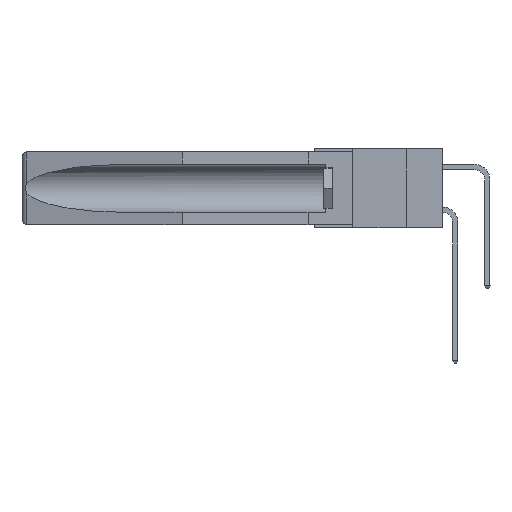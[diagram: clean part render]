
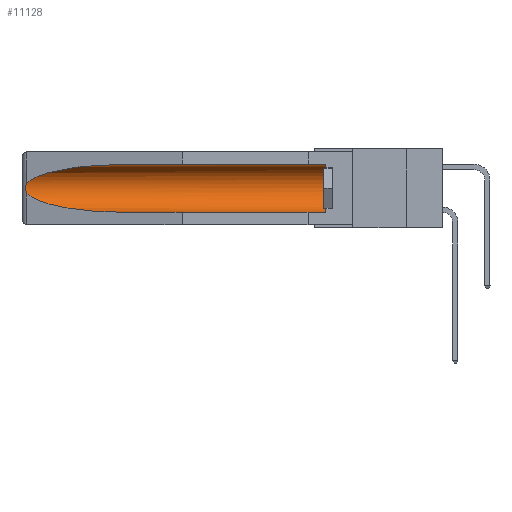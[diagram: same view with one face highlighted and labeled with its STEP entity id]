
A CAD part, left-side view. The second image highlights one B-rep face of the part: STEP entity #11128.
In plain terms, the highlighted cylindrical face has radius 2.857 mm (diameter 5.715 mm), a partial arc.
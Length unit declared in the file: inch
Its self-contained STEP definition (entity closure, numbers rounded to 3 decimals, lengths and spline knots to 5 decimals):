
#274 = DIRECTION ( 'NONE',  ( 0., 1., 0. ) ) ;
#505 = CARTESIAN_POINT ( 'NONE',  ( 0.26654, 1.53092, -0.15636 ) ) ;
#979 = CARTESIAN_POINT ( 'NONE',  ( 0.155, 1.07973, -0.059 ) ) ;
#1048 = ORIENTED_EDGE ( 'NONE', *, *, #12616, .F. ) ;
#1132 = CARTESIAN_POINT ( 'NONE',  ( 0.26597, 1.5296, -0.19026 ) ) ;
#1247 = CARTESIAN_POINT ( 'NONE',  ( 0.25451, 1.48313, -0.09465 ) ) ;
#1289 = DIRECTION ( 'NONE',  ( 0., 1., 0. ) ) ;
#1413 = CARTESIAN_POINT ( 'NONE',  ( 0.26537, 1.52718, -0.19328 ) ) ;
#1963 = B_SPLINE_CURVE_WITH_KNOTS ( 'NONE', 3,
 ( #6888, #18015, #505, #19783, #10522, #9368, #10989, #17308, #1132, #1413 ),
 .UNSPECIFIED., .F., .F.,
 ( 4, 2, 2, 2, 4 ),
 ( 0., 0.00029, 0.00058, 0.00087, 0.00117 ),
 .UNSPECIFIED. ) ;
#1995 = VERTEX_POINT ( 'NONE', #18974 ) ;
#2083 = EDGE_CURVE ( 'NONE', #9188, #8213, #16844, .T. ) ;
#2129 = CARTESIAN_POINT ( 'NONE',  ( 0.155, 1.07973, -0.284 ) ) ;
#3179 = EDGE_CURVE ( 'NONE', #16438, #1995, #3312, .T. ) ;
#3312 = CIRCLE ( 'NONE', #11565, 0.1125 ) ;
#3377 = CARTESIAN_POINT ( 'NONE',  ( 0.155, -0.30754, -0.1715 ) ) ;
#3535 = CARTESIAN_POINT ( 'NONE',  ( 0.21114, 1.30732, -0.284 ) ) ;
#3674 = CARTESIAN_POINT ( 'NONE',  ( 0.26537, 1.52718, -0.19328 ) ) ;
#5363 = LINE ( 'NONE', #9934, #17664 ) ;
#6613 = ORIENTED_EDGE ( 'NONE', *, *, #2083, .T. ) ;
#6749 = CYLINDRICAL_SURFACE ( 'NONE', #13404, 0.1125 ) ;
#6888 = CARTESIAN_POINT ( 'NONE',  ( 0.26537, 1.52718, -0.14972 ) ) ;
#6999 = EDGE_CURVE ( 'NONE', #15827, #7365, #18408, .T. ) ;
#7365 = VERTEX_POINT ( 'NONE', #19484 ) ;
#7812 = CARTESIAN_POINT ( 'NONE',  ( 0.155, 0.126, -0.1715 ) ) ;
#7888 = DIRECTION ( 'NONE',  ( 0., -1., 0. ) ) ;
#8213 = VERTEX_POINT ( 'NONE', #15224 ) ;
#8475 = FACE_OUTER_BOUND ( 'NONE', #11126, .T. ) ;
#8917 = CARTESIAN_POINT ( 'NONE',  ( 0.155, 0.126, -0.284 ) ) ;
#9064 = ORIENTED_EDGE ( 'NONE', *, *, #6999, .T. ) ;
#9072 = CARTESIAN_POINT ( 'NONE',  ( 0.21114, 1.30732, -0.059 ) ) ;
#9118 = CARTESIAN_POINT ( 'NONE',  ( 0.155, -0.30754, -0.284 ) ) ;
#9188 = VERTEX_POINT ( 'NONE', #16502 ) ;
#9368 = CARTESIAN_POINT ( 'NONE',  ( 0.2675, 1.53308, -0.17534 ) ) ;
#9403 = ORIENTED_EDGE ( 'NONE', *, *, #3179, .T. ) ;
#9411 = DIRECTION ( 'NONE',  ( 0., 0., 1. ) ) ;
#9858 = ORIENTED_EDGE ( 'NONE', *, *, #10091, .T. ) ;
#9934 = CARTESIAN_POINT ( 'NONE',  ( 0.155, -0.30754, -0.059 ) ) ;
#10091 = EDGE_CURVE ( 'NONE', #7365, #9188, #1963, .T. ) ;
#10522 = CARTESIAN_POINT ( 'NONE',  ( 0.2675, 1.53308, -0.16763 ) ) ;
#10989 = CARTESIAN_POINT ( 'NONE',  ( 0.2673, 1.53269, -0.17917 ) ) ;
#11126 = EDGE_LOOP ( 'NONE', ( #9064, #9858, #6613, #1048, #9403, #17494 ) ) ;
#11128 = ADVANCED_FACE ( 'NONE', ( #8475 ), #6749, .F. ) ;
#11535 = DIRECTION ( 'NONE',  ( 0., 1., 0. ) ) ;
#11565 = AXIS2_PLACEMENT_3D ( 'NONE', #7812, #7888, #9411 ) ;
#11685 = CARTESIAN_POINT ( 'NONE',  ( 0.25451, 1.48313, -0.24835 ) ) ;
#12213 = CARTESIAN_POINT ( 'NONE',  ( 0.26537, 1.52718, -0.14972 ) ) ;
#12616 = EDGE_CURVE ( 'NONE', #16438, #8213, #19848, .T. ) ;
#13202 = DIRECTION ( 'NONE',  ( 0., 0., 1. ) ) ;
#13235 = EDGE_CURVE ( 'NONE', #1995, #15827, #5363, .T. ) ;
#13404 = AXIS2_PLACEMENT_3D ( 'NONE', #3377, #274, #13202 ) ;
#15224 = CARTESIAN_POINT ( 'NONE',  ( 0.155, 1.07973, -0.284 ) ) ;
#15322 = VECTOR ( 'NONE', #1289, 39.37008 ) ;
#15827 = VERTEX_POINT ( 'NONE', #15912 ) ;
#15912 = CARTESIAN_POINT ( 'NONE',  ( 0.155, 1.07973, -0.059 ) ) ;
#16438 = VERTEX_POINT ( 'NONE', #8917 ) ;
#16502 = CARTESIAN_POINT ( 'NONE',  ( 0.26537, 1.52718, -0.19328 ) ) ;
#16844 =( BOUNDED_CURVE ( )  B_SPLINE_CURVE ( 3, ( #3674, #11685, #3535, #2129 ),
 .UNSPECIFIED., .F., .F. ) 
 B_SPLINE_CURVE_WITH_KNOTS ( ( 4, 4 ),
 ( 0.1948, 1.5708 ),
 .UNSPECIFIED. ) 
 CURVE ( )  GEOMETRIC_REPRESENTATION_ITEM ( )  RATIONAL_B_SPLINE_CURVE ( ( 1., 0.848, 0.848, 1. ) ) 
 REPRESENTATION_ITEM ( '' )  );
#17308 = CARTESIAN_POINT ( 'NONE',  ( 0.26655, 1.53094, -0.18657 ) ) ;
#17494 = ORIENTED_EDGE ( 'NONE', *, *, #13235, .T. ) ;
#17664 = VECTOR ( 'NONE', #11535, 39.37008 ) ;
#18015 = CARTESIAN_POINT ( 'NONE',  ( 0.26597, 1.52961, -0.15275 ) ) ;
#18408 =( BOUNDED_CURVE ( )  B_SPLINE_CURVE ( 3, ( #979, #9072, #1247, #12213 ),
 .UNSPECIFIED., .F., .F. ) 
 B_SPLINE_CURVE_WITH_KNOTS ( ( 4, 4 ),
 ( 4.71239, 6.08839 ),
 .UNSPECIFIED. ) 
 CURVE ( )  GEOMETRIC_REPRESENTATION_ITEM ( )  RATIONAL_B_SPLINE_CURVE ( ( 1., 0.848, 0.848, 1. ) ) 
 REPRESENTATION_ITEM ( '' )  );
#18974 = CARTESIAN_POINT ( 'NONE',  ( 0.155, 0.126, -0.059 ) ) ;
#19484 = CARTESIAN_POINT ( 'NONE',  ( 0.26537, 1.52718, -0.14972 ) ) ;
#19783 = CARTESIAN_POINT ( 'NONE',  ( 0.2673, 1.5327, -0.16383 ) ) ;
#19848 = LINE ( 'NONE', #9118, #15322 ) ;
